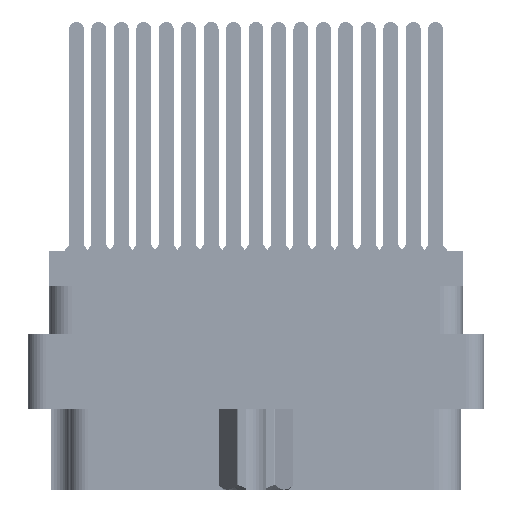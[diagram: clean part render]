
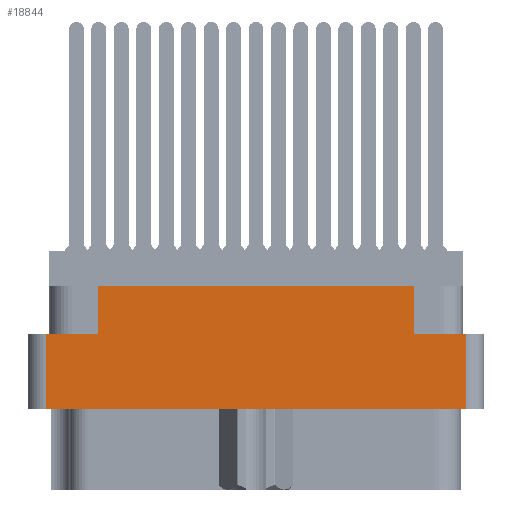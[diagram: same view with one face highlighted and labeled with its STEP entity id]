
A CAD part, left-side view. The second image highlights one B-rep face of the part: STEP entity #18844.
In plain terms, the highlighted planar face has unit normal (-1, 0, 0).
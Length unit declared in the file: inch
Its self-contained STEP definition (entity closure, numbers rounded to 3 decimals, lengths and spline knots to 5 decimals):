
#859 = VERTEX_POINT ( 'NONE', #90965 ) ;
#6401 = EDGE_CURVE ( 'NONE', #25299, #859, #89316, .T. ) ;
#7769 = VERTEX_POINT ( 'NONE', #46815 ) ;
#11211 = DIRECTION ( 'NONE',  ( -1., 0., 0. ) ) ;
#13300 = CARTESIAN_POINT ( 'NONE',  ( -1.375, 0.7005, -0.277 ) ) ;
#15323 = VECTOR ( 'NONE', #101687, 39.37008 ) ;
#15866 = DIRECTION ( 'NONE',  ( 0., -1., 0. ) ) ;
#16377 = ORIENTED_EDGE ( 'NONE', *, *, #54475, .T. ) ;
#16610 = LINE ( 'NONE', #83560, #15323 ) ;
#18829 = VECTOR ( 'NONE', #55611, 39.37008 ) ;
#18844 = ADVANCED_FACE ( 'NONE', ( #24319 ), #43733, .T. ) ;
#18999 = VECTOR ( 'NONE', #15866, 39.37008 ) ;
#19483 = VERTEX_POINT ( 'NONE', #19493 ) ;
#19493 = CARTESIAN_POINT ( 'NONE',  ( -1.375, -0.7005, -0.529 ) ) ;
#22125 = AXIS2_PLACEMENT_3D ( 'NONE', #82343, #11211, #26585 ) ;
#23376 = VERTEX_POINT ( 'NONE', #81372 ) ;
#23880 = CARTESIAN_POINT ( 'NONE',  ( -1.375, 0.7625, -0.117 ) ) ;
#24319 = FACE_OUTER_BOUND ( 'NONE', #39701, .T. ) ;
#25299 = VERTEX_POINT ( 'NONE', #13300 ) ;
#26585 = DIRECTION ( 'NONE',  ( 0., 0., 1. ) ) ;
#31061 = VECTOR ( 'NONE', #88285, 39.37008 ) ;
#31109 = VECTOR ( 'NONE', #73643, 39.37008 ) ;
#35894 = ORIENTED_EDGE ( 'NONE', *, *, #6401, .F. ) ;
#38610 = DIRECTION ( 'NONE',  ( 0., 1., 0. ) ) ;
#39212 = LINE ( 'NONE', #79424, #76775 ) ;
#39701 = EDGE_LOOP ( 'NONE', ( #35894, #76054, #89504, #16377, #47355, #77389, #87007, #98404 ) ) ;
#40300 = LINE ( 'NONE', #23880, #18999 ) ;
#40895 = CARTESIAN_POINT ( 'NONE',  ( -1.375, 0.5285, -0.117 ) ) ;
#43163 = VECTOR ( 'NONE', #38610, 39.37008 ) ;
#43733 = PLANE ( 'NONE',  #22125 ) ;
#44829 = LINE ( 'NONE', #79849, #31061 ) ;
#46664 = VECTOR ( 'NONE', #52019, 39.37008 ) ;
#46815 = CARTESIAN_POINT ( 'NONE',  ( -1.375, 0.7005, -0.529 ) ) ;
#47355 = ORIENTED_EDGE ( 'NONE', *, *, #58123, .F. ) ;
#47549 = DIRECTION ( 'NONE',  ( 0., -1., 0. ) ) ;
#48036 = CARTESIAN_POINT ( 'NONE',  ( -1.375, 0., -0.529 ) ) ;
#48432 = CARTESIAN_POINT ( 'NONE',  ( -1.375, -0.7005, -0.798 ) ) ;
#52019 = DIRECTION ( 'NONE',  ( 0., -1., 0. ) ) ;
#54351 = CARTESIAN_POINT ( 'NONE',  ( -1.375, -0.7005, -0.277 ) ) ;
#54475 = EDGE_CURVE ( 'NONE', #19483, #102400, #72572, .T. ) ;
#55611 = DIRECTION ( 'NONE',  ( 0., 0., 1. ) ) ;
#56892 = EDGE_CURVE ( 'NONE', #19483, #7769, #94568, .T. ) ;
#58123 = EDGE_CURVE ( 'NONE', #63444, #102400, #39212, .T. ) ;
#58444 = EDGE_CURVE ( 'NONE', #63444, #23376, #16610, .T. ) ;
#59126 = EDGE_CURVE ( 'NONE', #85761, #23376, #40300, .T. ) ;
#63232 = CARTESIAN_POINT ( 'NONE',  ( -1.375, -0.5285, -0.277 ) ) ;
#63444 = VERTEX_POINT ( 'NONE', #63232 ) ;
#68128 = CARTESIAN_POINT ( 'NONE',  ( -1.375, 0., -0.277 ) ) ;
#68947 = EDGE_CURVE ( 'NONE', #859, #85761, #96504, .T. ) ;
#70148 = EDGE_CURVE ( 'NONE', #25299, #7769, #44829, .T. ) ;
#71080 = CARTESIAN_POINT ( 'NONE',  ( -1.375, 0.5285, -0.277 ) ) ;
#72572 = LINE ( 'NONE', #48432, #31109 ) ;
#73643 = DIRECTION ( 'NONE',  ( 0., 0., 1. ) ) ;
#76054 = ORIENTED_EDGE ( 'NONE', *, *, #70148, .T. ) ;
#76775 = VECTOR ( 'NONE', #47549, 39.37008 ) ;
#77389 = ORIENTED_EDGE ( 'NONE', *, *, #58444, .T. ) ;
#79424 = CARTESIAN_POINT ( 'NONE',  ( -1.375, 0., -0.277 ) ) ;
#79849 = CARTESIAN_POINT ( 'NONE',  ( -1.375, 0.7005, -0.798 ) ) ;
#81372 = CARTESIAN_POINT ( 'NONE',  ( -1.375, -0.5285, -0.117 ) ) ;
#82343 = CARTESIAN_POINT ( 'NONE',  ( -1.375, -0.7625, -0.798 ) ) ;
#83560 = CARTESIAN_POINT ( 'NONE',  ( -1.375, -0.5285, -0.277 ) ) ;
#85761 = VERTEX_POINT ( 'NONE', #40895 ) ;
#87007 = ORIENTED_EDGE ( 'NONE', *, *, #59126, .F. ) ;
#88285 = DIRECTION ( 'NONE',  ( 0., 0., -1. ) ) ;
#89316 = LINE ( 'NONE', #68128, #46664 ) ;
#89504 = ORIENTED_EDGE ( 'NONE', *, *, #56892, .F. ) ;
#90965 = CARTESIAN_POINT ( 'NONE',  ( -1.375, 0.5285, -0.277 ) ) ;
#94568 = LINE ( 'NONE', #48036, #43163 ) ;
#96504 = LINE ( 'NONE', #71080, #18829 ) ;
#98404 = ORIENTED_EDGE ( 'NONE', *, *, #68947, .F. ) ;
#101687 = DIRECTION ( 'NONE',  ( 0., 0., 1. ) ) ;
#102400 = VERTEX_POINT ( 'NONE', #54351 ) ;
